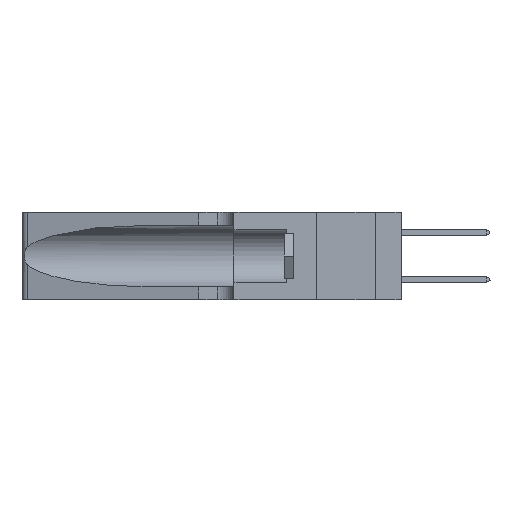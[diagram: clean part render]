
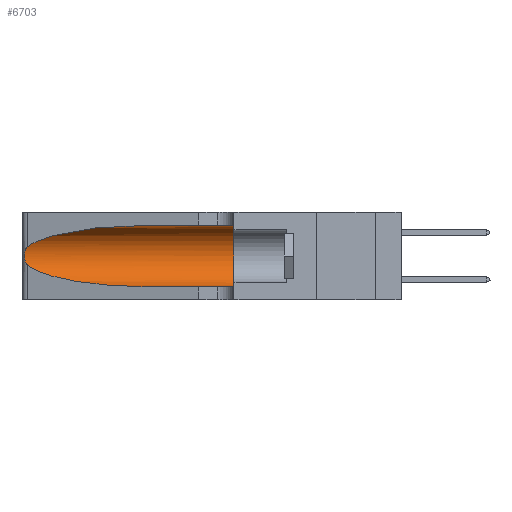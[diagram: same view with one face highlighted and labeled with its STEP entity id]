
A CAD part, left-side view. The second image highlights one B-rep face of the part: STEP entity #6703.
In plain terms, the highlighted cylindrical face has radius 3.308 mm (diameter 6.617 mm), a partial arc.
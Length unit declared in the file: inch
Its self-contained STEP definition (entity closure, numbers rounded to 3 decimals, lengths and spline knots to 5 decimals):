
#11 = ORIENTED_EDGE ( 'NONE', *, *, #14520, .T. ) ;
#198 = EDGE_LOOP ( 'NONE', ( #7387, #819, #6580, #11, #27114, #20170 ) ) ;
#737 = CARTESIAN_POINT ( 'NONE',  ( 0.25639, 1.23186, 0.15144 ) ) ;
#819 = ORIENTED_EDGE ( 'NONE', *, *, #3868, .T. ) ;
#1084 = CARTESIAN_POINT ( 'NONE',  ( 0.25487, 1.22718, 0.14631 ) ) ;
#1246 = VERTEX_POINT ( 'NONE', #2835 ) ;
#1600 = CARTESIAN_POINT ( 'NONE',  ( 0.25487, 1.22718, 0.14631 ) ) ;
#2090 = AXIS2_PLACEMENT_3D ( 'NONE', #27137, #10485, #27135 ) ;
#2740 = CARTESIAN_POINT ( 'NONE',  ( 0.25789, 1.23486, 0.15765 ) ) ;
#2835 = CARTESIAN_POINT ( 'NONE',  ( 0.1305, 0.35, 0.31525 ) ) ;
#2855 = CARTESIAN_POINT ( 'NONE',  ( 0.1305, 1.61858, 0.31525 ) ) ;
#3290 = B_SPLINE_CURVE_WITH_KNOTS ( 'NONE', 3,
 ( #26997, #22909, #14664, #4486, #12870, #9213, #7683, #11119, #13640, #20985, #2740, #737, #9853, #1084 ),
 .UNSPECIFIED., .F., .F.,
 ( 4, 2, 2, 2, 2, 2, 4 ),
 ( 0., 0.00027, 0.00053, 0.00107, 0.0016, 0.00187, 0.00214 ),
 .UNSPECIFIED. ) ;
#3868 = EDGE_CURVE ( 'NONE', #13463, #8005, #3290, .T. ) ;
#3965 = CARTESIAN_POINT ( 'NONE',  ( 0.1305, 0.72297, 0.05475 ) ) ;
#4126 = VERTEX_POINT ( 'NONE', #10248 ) ;
#4151 = CARTESIAN_POINT ( 'NONE',  ( 0.1305, 0.72297, 0.31525 ) ) ;
#4237 = CARTESIAN_POINT ( 'NONE',  ( 0.25487, 1.22718, 0.22369 ) ) ;
#4486 = CARTESIAN_POINT ( 'NONE',  ( 0.25787, 1.23484, 0.2124 ) ) ;
#4664 = AXIS2_PLACEMENT_3D ( 'NONE', #25966, #4898, #13168 ) ;
#4861 = VECTOR ( 'NONE', #17742, 39.37008 ) ;
#4898 = DIRECTION ( 'NONE',  ( 0., -1., 0. ) ) ;
#6580 = ORIENTED_EDGE ( 'NONE', *, *, #22740, .T. ) ;
#6703 = ADVANCED_FACE ( 'NONE', ( #19936 ), #23926, .F. ) ;
#7220 = DIRECTION ( 'NONE',  ( 0., -1., 0. ) ) ;
#7387 = ORIENTED_EDGE ( 'NONE', *, *, #18853, .T. ) ;
#7683 = CARTESIAN_POINT ( 'NONE',  ( 0.26075, 1.23896, 0.19203 ) ) ;
#8005 = VERTEX_POINT ( 'NONE', #24238 ) ;
#8340 = CARTESIAN_POINT ( 'NONE',  ( 0.18966, 0.96281, 0.31525 ) ) ;
#8374 = EDGE_CURVE ( 'NONE', #4126, #1246, #10504, .T. ) ;
#9213 = CARTESIAN_POINT ( 'NONE',  ( 0.26018, 1.23835, 0.19895 ) ) ;
#9447 = CARTESIAN_POINT ( 'NONE',  ( 0.1305, 0.35, 0.05475 ) ) ;
#9853 = CARTESIAN_POINT ( 'NONE',  ( 0.25555, 1.22993, 0.14849 ) ) ;
#10095 = CARTESIAN_POINT ( 'NONE',  ( 0.2373, 1.15595, 0.08982 ) ) ;
#10248 = CARTESIAN_POINT ( 'NONE',  ( 0.1305, 0.72297, 0.31525 ) ) ;
#10485 = DIRECTION ( 'NONE',  ( 0., 1., 0. ) ) ;
#10504 = LINE ( 'NONE', #2855, #4861 ) ;
#11119 = CARTESIAN_POINT ( 'NONE',  ( 0.26075, 1.23896, 0.178 ) ) ;
#11734 = VERTEX_POINT ( 'NONE', #9447 ) ;
#12870 = CARTESIAN_POINT ( 'NONE',  ( 0.25854, 1.2359, 0.20912 ) ) ;
#13168 = DIRECTION ( 'NONE',  ( 0., 0., -1. ) ) ;
#13463 = VERTEX_POINT ( 'NONE', #19973 ) ;
#13640 = CARTESIAN_POINT ( 'NONE',  ( 0.26017, 1.23833, 0.17102 ) ) ;
#14120 = VECTOR ( 'NONE', #7220, 39.37008 ) ;
#14520 = EDGE_CURVE ( 'NONE', #23877, #11734, #16117, .T. ) ;
#14664 = CARTESIAN_POINT ( 'NONE',  ( 0.25639, 1.23184, 0.21858 ) ) ;
#16117 = LINE ( 'NONE', #22506, #14120 ) ;
#17034 = CARTESIAN_POINT ( 'NONE',  ( 0.2373, 1.15595, 0.28018 ) ) ;
#17742 = DIRECTION ( 'NONE',  ( 0., -1., 0. ) ) ;
#18632 =( BOUNDED_CURVE ( )  B_SPLINE_CURVE ( 3, ( #4151, #8340, #17034, #4237 ),
 .UNSPECIFIED., .F., .T. ) 
 B_SPLINE_CURVE_WITH_KNOTS ( ( 4, 4 ),
 ( 1.5708, 2.84003 ),
 .UNSPECIFIED. ) 
 CURVE ( )  GEOMETRIC_REPRESENTATION_ITEM ( )  RATIONAL_B_SPLINE_CURVE ( ( 1., 0.87, 0.87, 1. ) ) 
 REPRESENTATION_ITEM ( '' )  );
#18853 = EDGE_CURVE ( 'NONE', #4126, #13463, #18632, .T. ) ;
#18867 = EDGE_CURVE ( 'NONE', #1246, #11734, #22554, .T. ) ;
#19936 = FACE_OUTER_BOUND ( 'NONE', #198, .T. ) ;
#19973 = CARTESIAN_POINT ( 'NONE',  ( 0.25487, 1.22718, 0.22369 ) ) ;
#20170 = ORIENTED_EDGE ( 'NONE', *, *, #8374, .F. ) ;
#20985 = CARTESIAN_POINT ( 'NONE',  ( 0.25856, 1.23593, 0.16098 ) ) ;
#22506 = CARTESIAN_POINT ( 'NONE',  ( 0.1305, 1.61858, 0.05475 ) ) ;
#22554 = CIRCLE ( 'NONE', #2090, 0.13025 ) ;
#22740 = EDGE_CURVE ( 'NONE', #8005, #23877, #25584, .T. ) ;
#22909 = CARTESIAN_POINT ( 'NONE',  ( 0.25555, 1.22994, 0.2215 ) ) ;
#23877 = VERTEX_POINT ( 'NONE', #26376 ) ;
#23926 = CYLINDRICAL_SURFACE ( 'NONE', #4664, 0.13025 ) ;
#24238 = CARTESIAN_POINT ( 'NONE',  ( 0.25487, 1.22718, 0.14631 ) ) ;
#25584 =( BOUNDED_CURVE ( )  B_SPLINE_CURVE ( 3, ( #1600, #10095, #27211, #3965 ),
 .UNSPECIFIED., .F., .F. ) 
 B_SPLINE_CURVE_WITH_KNOTS ( ( 4, 4 ),
 ( 3.44316, 4.71239 ),
 .UNSPECIFIED. ) 
 CURVE ( )  GEOMETRIC_REPRESENTATION_ITEM ( )  RATIONAL_B_SPLINE_CURVE ( ( 1., 0.87, 0.87, 1. ) ) 
 REPRESENTATION_ITEM ( '' )  );
#25966 = CARTESIAN_POINT ( 'NONE',  ( 0.1305, 1.61858, 0.185 ) ) ;
#26376 = CARTESIAN_POINT ( 'NONE',  ( 0.1305, 0.72297, 0.05475 ) ) ;
#26997 = CARTESIAN_POINT ( 'NONE',  ( 0.25487, 1.22718, 0.22369 ) ) ;
#27114 = ORIENTED_EDGE ( 'NONE', *, *, #18867, .F. ) ;
#27135 = DIRECTION ( 'NONE',  ( 0., 0., 1. ) ) ;
#27137 = CARTESIAN_POINT ( 'NONE',  ( 0.1305, 0.35, 0.185 ) ) ;
#27211 = CARTESIAN_POINT ( 'NONE',  ( 0.18966, 0.96281, 0.05475 ) ) ;
